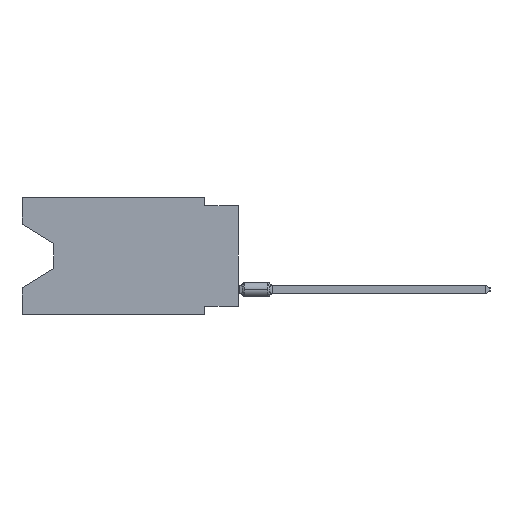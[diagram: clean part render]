
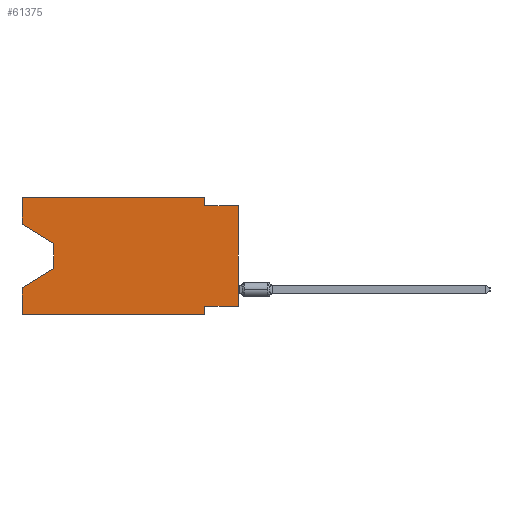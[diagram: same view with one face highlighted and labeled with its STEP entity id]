
A CAD part, left-side view. The second image highlights one B-rep face of the part: STEP entity #61375.
In plain terms, the highlighted planar face has unit normal (-1, 0, 0).
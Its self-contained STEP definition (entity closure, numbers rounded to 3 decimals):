
#317 = CARTESIAN_POINT ( 'NONE',  ( 0., 16.383, -2.038 ) ) ;
#919 = VERTEX_POINT ( 'NONE', #47137 ) ;
#1436 = EDGE_CURVE ( 'NONE', #7682, #40748, #12849, .T. ) ;
#5620 = VECTOR ( 'NONE', #20363, 1000. ) ;
#5971 = FACE_OUTER_BOUND ( 'NONE', #31411, .T. ) ;
#7682 = VERTEX_POINT ( 'NONE', #317 ) ;
#8161 = AXIS2_PLACEMENT_3D ( 'NONE', #41720, #62111, #57098 ) ;
#8342 = ORIENTED_EDGE ( 'NONE', *, *, #64363, .F. ) ;
#8715 = LINE ( 'NONE', #44464, #52683 ) ;
#8752 = LINE ( 'NONE', #29788, #30908 ) ;
#8790 = CARTESIAN_POINT ( 'NONE',  ( 0., 2.54, -0.635 ) ) ;
#9658 = CARTESIAN_POINT ( 'NONE',  ( 0., 16.383, 0. ) ) ;
#11433 = ORIENTED_EDGE ( 'NONE', *, *, #54894, .T. ) ;
#12757 = VECTOR ( 'NONE', #38233, 1000. ) ;
#12849 = LINE ( 'NONE', #37885, #42696 ) ;
#13453 = VECTOR ( 'NONE', #56905, 1000. ) ;
#14408 = DIRECTION ( 'NONE',  ( 0., 0., -1. ) ) ;
#16442 = CARTESIAN_POINT ( 'NONE',  ( 0., 16.383, -8.89 ) ) ;
#19435 = CARTESIAN_POINT ( 'NONE',  ( 0., 2.54, 0. ) ) ;
#19925 = ORIENTED_EDGE ( 'NONE', *, *, #21274, .F. ) ;
#20011 = VERTEX_POINT ( 'NONE', #16442 ) ;
#20024 = CARTESIAN_POINT ( 'NONE',  ( 0., 13.97, -5.385 ) ) ;
#20363 = DIRECTION ( 'NONE',  ( 0., 0.855, -0.519 ) ) ;
#20421 = ORIENTED_EDGE ( 'NONE', *, *, #1436, .F. ) ;
#20694 = LINE ( 'NONE', #9658, #51239 ) ;
#21274 = EDGE_CURVE ( 'NONE', #919, #21694, #23259, .T. ) ;
#21694 = VERTEX_POINT ( 'NONE', #26544 ) ;
#23259 = LINE ( 'NONE', #26945, #54472 ) ;
#23375 = CARTESIAN_POINT ( 'NONE',  ( 0., 13.97, -5.385 ) ) ;
#23523 = CARTESIAN_POINT ( 'NONE',  ( 0., 16.383, 0. ) ) ;
#25083 = EDGE_CURVE ( 'NONE', #56493, #65448, #26368, .T. ) ;
#26109 = CARTESIAN_POINT ( 'NONE',  ( 0., 16.383, 0. ) ) ;
#26368 = LINE ( 'NONE', #20024, #5620 ) ;
#26385 = PLANE ( 'NONE',  #8161 ) ;
#26544 = CARTESIAN_POINT ( 'NONE',  ( 0., 2.54, -8.255 ) ) ;
#26677 = VERTEX_POINT ( 'NONE', #46144 ) ;
#26765 = LINE ( 'NONE', #26109, #62946 ) ;
#26809 = EDGE_CURVE ( 'NONE', #20011, #65448, #20694, .T. ) ;
#26945 = CARTESIAN_POINT ( 'NONE',  ( 0., 0., -8.255 ) ) ;
#28762 = ORIENTED_EDGE ( 'NONE', *, *, #25083, .T. ) ;
#29696 = VERTEX_POINT ( 'NONE', #44868 ) ;
#29788 = CARTESIAN_POINT ( 'NONE',  ( 0., 0., -0.635 ) ) ;
#30506 = LINE ( 'NONE', #61896, #42822 ) ;
#30908 = VECTOR ( 'NONE', #60192, 1000. ) ;
#31411 = EDGE_LOOP ( 'NONE', ( #58694, #59127, #28762, #51895, #11433, #59390, #19925, #39102, #42306, #62899, #8342, #20421 ) ) ;
#31838 = LINE ( 'NONE', #56232, #13453 ) ;
#32161 = CARTESIAN_POINT ( 'NONE',  ( 0., 13.97, -3.505 ) ) ;
#34410 = VECTOR ( 'NONE', #50462, 1000. ) ;
#36177 = DIRECTION ( 'NONE',  ( 0., 0., -1. ) ) ;
#37885 = CARTESIAN_POINT ( 'NONE',  ( 0., 16.383, 0. ) ) ;
#38233 = DIRECTION ( 'NONE',  ( 0., 0., 1. ) ) ;
#39102 = ORIENTED_EDGE ( 'NONE', *, *, #47085, .T. ) ;
#39712 = DIRECTION ( 'NONE',  ( 0., 0., 1. ) ) ;
#40088 = VERTEX_POINT ( 'NONE', #32161 ) ;
#40748 = VERTEX_POINT ( 'NONE', #23523 ) ;
#40806 = VERTEX_POINT ( 'NONE', #8790 ) ;
#41163 = CARTESIAN_POINT ( 'NONE',  ( 0., 16.383, -6.852 ) ) ;
#41720 = CARTESIAN_POINT ( 'NONE',  ( 0., 16.383, 0. ) ) ;
#41765 = VERTEX_POINT ( 'NONE', #48090 ) ;
#42306 = ORIENTED_EDGE ( 'NONE', *, *, #47574, .F. ) ;
#42595 = CARTESIAN_POINT ( 'NONE',  ( 0., 0., 0. ) ) ;
#42696 = VECTOR ( 'NONE', #53587, 1000. ) ;
#42822 = VECTOR ( 'NONE', #36177, 1000. ) ;
#43794 = LINE ( 'NONE', #64163, #34410 ) ;
#44464 = CARTESIAN_POINT ( 'NONE',  ( 0., 16.383, -2.038 ) ) ;
#44868 = CARTESIAN_POINT ( 'NONE',  ( 0., 2.54, -8.89 ) ) ;
#46144 = CARTESIAN_POINT ( 'NONE',  ( 0., 0., -0.635 ) ) ;
#47085 = EDGE_CURVE ( 'NONE', #919, #26677, #47972, .T. ) ;
#47137 = CARTESIAN_POINT ( 'NONE',  ( 0., 0., -8.255 ) ) ;
#47574 = EDGE_CURVE ( 'NONE', #40806, #26677, #8752, .T. ) ;
#47972 = LINE ( 'NONE', #42595, #12757 ) ;
#48090 = CARTESIAN_POINT ( 'NONE',  ( 0., 2.54, 0. ) ) ;
#48651 = DIRECTION ( 'NONE',  ( 0., 1., 0. ) ) ;
#50462 = DIRECTION ( 'NONE',  ( 0., -1., 0. ) ) ;
#51239 = VECTOR ( 'NONE', #39712, 1000. ) ;
#51895 = ORIENTED_EDGE ( 'NONE', *, *, #26809, .F. ) ;
#52683 = VECTOR ( 'NONE', #64833, 1000. ) ;
#53496 = VECTOR ( 'NONE', #14408, 1000. ) ;
#53587 = DIRECTION ( 'NONE',  ( 0., 0., 1. ) ) ;
#53713 = EDGE_CURVE ( 'NONE', #41765, #40806, #54820, .T. ) ;
#54472 = VECTOR ( 'NONE', #48651, 1000. ) ;
#54820 = LINE ( 'NONE', #19435, #53496 ) ;
#54894 = EDGE_CURVE ( 'NONE', #20011, #29696, #43794, .T. ) ;
#56232 = CARTESIAN_POINT ( 'NONE',  ( 0., 2.54, -8.89 ) ) ;
#56313 = EDGE_CURVE ( 'NONE', #7682, #40088, #8715, .T. ) ;
#56493 = VERTEX_POINT ( 'NONE', #23375 ) ;
#56905 = DIRECTION ( 'NONE',  ( 0., 0., -1. ) ) ;
#57098 = DIRECTION ( 'NONE',  ( 0., 0., -1. ) ) ;
#57477 = DIRECTION ( 'NONE',  ( 0., -1., 0. ) ) ;
#58280 = EDGE_CURVE ( 'NONE', #21694, #29696, #31838, .T. ) ;
#58694 = ORIENTED_EDGE ( 'NONE', *, *, #56313, .T. ) ;
#59127 = ORIENTED_EDGE ( 'NONE', *, *, #62797, .T. ) ;
#59390 = ORIENTED_EDGE ( 'NONE', *, *, #58280, .F. ) ;
#60192 = DIRECTION ( 'NONE',  ( 0., -1., 0. ) ) ;
#61375 = ADVANCED_FACE ( 'NONE', ( #5971 ), #26385, .F. ) ;
#61896 = CARTESIAN_POINT ( 'NONE',  ( 0., 13.97, -3.505 ) ) ;
#62111 = DIRECTION ( 'NONE',  ( 1., 0., 0. ) ) ;
#62797 = EDGE_CURVE ( 'NONE', #40088, #56493, #30506, .T. ) ;
#62899 = ORIENTED_EDGE ( 'NONE', *, *, #53713, .F. ) ;
#62946 = VECTOR ( 'NONE', #57477, 1000. ) ;
#64163 = CARTESIAN_POINT ( 'NONE',  ( 0., 16.383, -8.89 ) ) ;
#64363 = EDGE_CURVE ( 'NONE', #40748, #41765, #26765, .T. ) ;
#64833 = DIRECTION ( 'NONE',  ( 0., -0.855, -0.519 ) ) ;
#65448 = VERTEX_POINT ( 'NONE', #41163 ) ;
